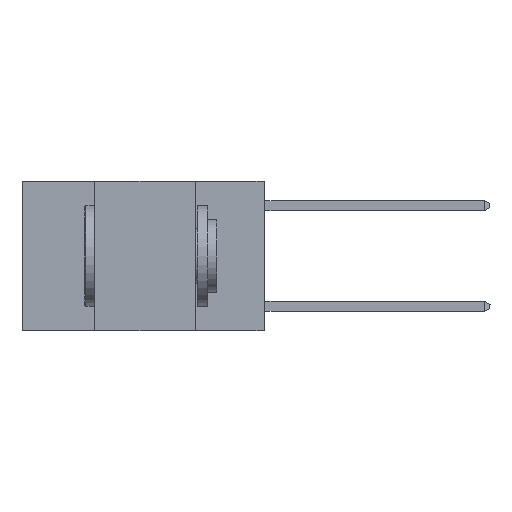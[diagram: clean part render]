
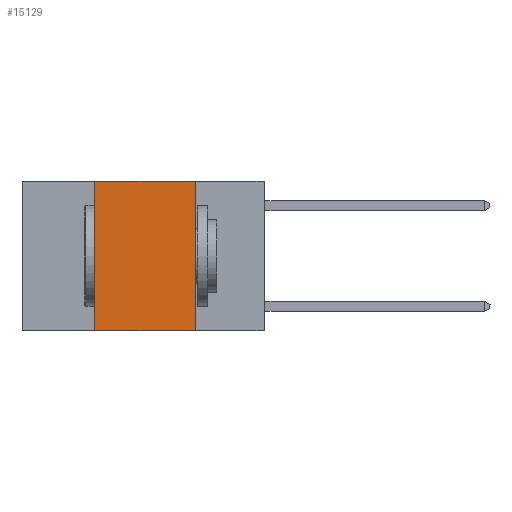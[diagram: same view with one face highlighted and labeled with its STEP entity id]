
A CAD part, left-side view. The second image highlights one B-rep face of the part: STEP entity #15129.
In plain terms, the highlighted planar face has unit normal (-1, 0, 0).
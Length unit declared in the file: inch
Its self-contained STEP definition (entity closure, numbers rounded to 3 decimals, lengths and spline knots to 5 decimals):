
#272 = CARTESIAN_POINT ( 'NONE',  ( 0., 0.17, 0. ) ) ;
#659 = FACE_OUTER_BOUND ( 'NONE', #9546, .T. ) ;
#1075 = CARTESIAN_POINT ( 'NONE',  ( 0., 0.6, 0. ) ) ;
#2051 = LINE ( 'NONE', #8740, #13074 ) ;
#3291 = DIRECTION ( 'NONE',  ( 0., 0., -1. ) ) ;
#3575 = CARTESIAN_POINT ( 'NONE',  ( 0., 0.42, 0. ) ) ;
#4426 = DIRECTION ( 'NONE',  ( 0., 0., -1. ) ) ;
#4893 = CARTESIAN_POINT ( 'NONE',  ( 0., 0.42, 0. ) ) ;
#6895 = VERTEX_POINT ( 'NONE', #272 ) ;
#8296 = CARTESIAN_POINT ( 'NONE',  ( 0., 0.42, -0.37 ) ) ;
#8304 = LINE ( 'NONE', #21993, #13450 ) ;
#8716 = EDGE_CURVE ( 'NONE', #15643, #6895, #8304, .T. ) ;
#8740 = CARTESIAN_POINT ( 'NONE',  ( 0., 0.6, -0.37 ) ) ;
#9546 = EDGE_LOOP ( 'NONE', ( #26943, #26952, #26376, #22372 ) ) ;
#10912 = LINE ( 'NONE', #3575, #22023 ) ;
#11332 = EDGE_CURVE ( 'NONE', #23241, #15643, #10912, .T. ) ;
#11804 = VECTOR ( 'NONE', #4426, 39.37008 ) ;
#13074 = VECTOR ( 'NONE', #19756, 39.37008 ) ;
#13184 = LINE ( 'NONE', #15441, #11804 ) ;
#13450 = VECTOR ( 'NONE', #17488, 39.37008 ) ;
#15129 = ADVANCED_FACE ( 'NONE', ( #659 ), #27633, .F. ) ;
#15441 = CARTESIAN_POINT ( 'NONE',  ( 0., 0.17, 0. ) ) ;
#15643 = VERTEX_POINT ( 'NONE', #4893 ) ;
#16507 = DIRECTION ( 'NONE',  ( 1., 0., 0. ) ) ;
#17488 = DIRECTION ( 'NONE',  ( 0., -1., 0. ) ) ;
#19756 = DIRECTION ( 'NONE',  ( 0., -1., 0. ) ) ;
#21993 = CARTESIAN_POINT ( 'NONE',  ( 0., 0.6, 0. ) ) ;
#22023 = VECTOR ( 'NONE', #25787, 39.37008 ) ;
#22372 = ORIENTED_EDGE ( 'NONE', *, *, #24947, .T. ) ;
#22711 = EDGE_CURVE ( 'NONE', #6895, #27627, #13184, .T. ) ;
#23241 = VERTEX_POINT ( 'NONE', #8296 ) ;
#24705 = AXIS2_PLACEMENT_3D ( 'NONE', #1075, #16507, #3291 ) ;
#24947 = EDGE_CURVE ( 'NONE', #23241, #27627, #2051, .T. ) ;
#25787 = DIRECTION ( 'NONE',  ( 0., 0., 1. ) ) ;
#26376 = ORIENTED_EDGE ( 'NONE', *, *, #11332, .F. ) ;
#26677 = CARTESIAN_POINT ( 'NONE',  ( 0., 0.17, -0.37 ) ) ;
#26943 = ORIENTED_EDGE ( 'NONE', *, *, #22711, .F. ) ;
#26952 = ORIENTED_EDGE ( 'NONE', *, *, #8716, .F. ) ;
#27627 = VERTEX_POINT ( 'NONE', #26677 ) ;
#27633 = PLANE ( 'NONE',  #24705 ) ;
